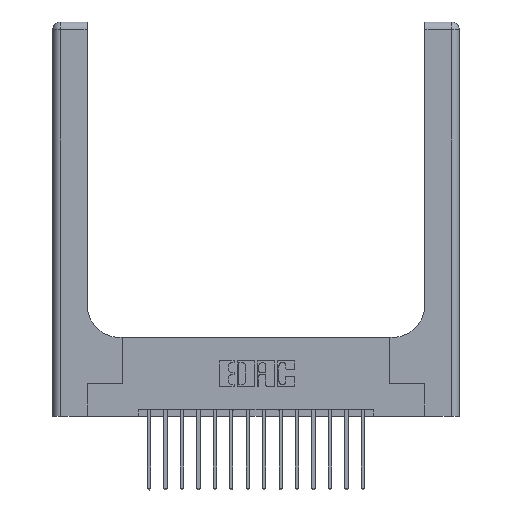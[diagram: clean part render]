
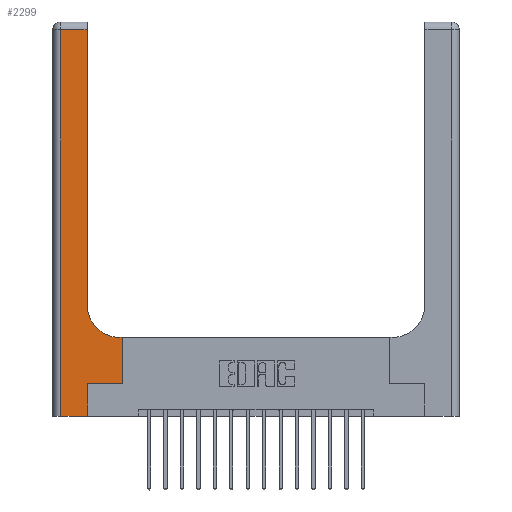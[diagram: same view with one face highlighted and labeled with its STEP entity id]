
A CAD part, top view. The second image highlights one B-rep face of the part: STEP entity #2299.
In plain terms, the highlighted planar face has unit normal (0, 0, 1).
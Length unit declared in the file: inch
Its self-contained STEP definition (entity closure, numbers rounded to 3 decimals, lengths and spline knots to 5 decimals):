
#27 = VERTEX_POINT ( 'NONE', #10364 ) ;
#259 = VERTEX_POINT ( 'NONE', #10660 ) ;
#442 = VECTOR ( 'NONE', #9737, 39.37008 ) ;
#500 = DIRECTION ( 'NONE',  ( 0., 1., 0. ) ) ;
#886 = CARTESIAN_POINT ( 'NONE',  ( 0.528, 0.25, 0.37 ) ) ;
#1867 = VERTEX_POINT ( 'NONE', #3295 ) ;
#1930 = VECTOR ( 'NONE', #9675, 39.37008 ) ;
#2299 = ADVANCED_FACE ( 'NONE', ( #17613 ), #8410, .F. ) ;
#2302 = ORIENTED_EDGE ( 'NONE', *, *, #12450, .T. ) ;
#2463 = CARTESIAN_POINT ( 'NONE',  ( 0., 0., 0.37 ) ) ;
#2522 = EDGE_CURVE ( 'NONE', #1867, #12474, #10802, .T. ) ;
#2961 = VECTOR ( 'NONE', #17435, 39.37008 ) ;
#3037 = ORIENTED_EDGE ( 'NONE', *, *, #3047, .T. ) ;
#3047 = EDGE_CURVE ( 'NONE', #12474, #259, #11000, .T. ) ;
#3295 = CARTESIAN_POINT ( 'NONE',  ( 0.528, 0.25, 0.37 ) ) ;
#3488 = ORIENTED_EDGE ( 'NONE', *, *, #9466, .T. ) ;
#3636 = DIRECTION ( 'NONE',  ( 1., 0., 0. ) ) ;
#3998 = AXIS2_PLACEMENT_3D ( 'NONE', #11201, #16624, #9816 ) ;
#4140 = ORIENTED_EDGE ( 'NONE', *, *, #8069, .T. ) ;
#4178 = CARTESIAN_POINT ( 'NONE',  ( 0.265, 0., 0.37 ) ) ;
#4180 = CARTESIAN_POINT ( 'NONE',  ( 0.265, 0.25, 0.37 ) ) ;
#4676 = ORIENTED_EDGE ( 'NONE', *, *, #7464, .T. ) ;
#4763 = LINE ( 'NONE', #4180, #16792 ) ;
#4932 = CARTESIAN_POINT ( 'NONE',  ( 0.51, 0.85, 0.37 ) ) ;
#5032 = CARTESIAN_POINT ( 'NONE',  ( 0.06, 2.94, 0.37 ) ) ;
#5108 = DIRECTION ( 'NONE',  ( 1., 0., 0. ) ) ;
#6316 = EDGE_CURVE ( 'NONE', #13782, #11043, #7664, .T. ) ;
#6340 = DIRECTION ( 'NONE',  ( 0., 0., -1. ) ) ;
#6595 = ORIENTED_EDGE ( 'NONE', *, *, #8855, .T. ) ;
#7026 = VERTEX_POINT ( 'NONE', #9818 ) ;
#7166 = LINE ( 'NONE', #11311, #1930 ) ;
#7381 = VECTOR ( 'NONE', #13764, 39.37008 ) ;
#7464 = EDGE_CURVE ( 'NONE', #11043, #27, #16376, .T. ) ;
#7519 = ORIENTED_EDGE ( 'NONE', *, *, #17191, .T. ) ;
#7664 = LINE ( 'NONE', #2463, #10480 ) ;
#8069 = EDGE_CURVE ( 'NONE', #7026, #16161, #7166, .T. ) ;
#8212 = ORIENTED_EDGE ( 'NONE', *, *, #2522, .T. ) ;
#8323 = DIRECTION ( 'NONE',  ( -1., 0., 0. ) ) ;
#8410 = PLANE ( 'NONE',  #3998 ) ;
#8855 = EDGE_CURVE ( 'NONE', #27, #1867, #4763, .T. ) ;
#9466 = EDGE_CURVE ( 'NONE', #16161, #13782, #15250, .T. ) ;
#9675 = DIRECTION ( 'NONE',  ( -1., 0., 0. ) ) ;
#9737 = DIRECTION ( 'NONE',  ( 0., 1., 0. ) ) ;
#9796 = ORIENTED_EDGE ( 'NONE', *, *, #6316, .T. ) ;
#9816 = DIRECTION ( 'NONE',  ( -1., 0., 0. ) ) ;
#9818 = CARTESIAN_POINT ( 'NONE',  ( 0.26, 2.94, 0.37 ) ) ;
#10044 = CARTESIAN_POINT ( 'NONE',  ( 0.528, 0.6, 0.37 ) ) ;
#10364 = CARTESIAN_POINT ( 'NONE',  ( 0.265, 0.25, 0.37 ) ) ;
#10480 = VECTOR ( 'NONE', #5108, 39.37008 ) ;
#10660 = CARTESIAN_POINT ( 'NONE',  ( 0.51, 0.6, 0.37 ) ) ;
#10802 = LINE ( 'NONE', #886, #2961 ) ;
#11000 = LINE ( 'NONE', #14005, #17596 ) ;
#11043 = VERTEX_POINT ( 'NONE', #4178 ) ;
#11201 = CARTESIAN_POINT ( 'NONE',  ( 0., 3., 0.37 ) ) ;
#11311 = CARTESIAN_POINT ( 'NONE',  ( 0., 2.94, 0.37 ) ) ;
#12450 = EDGE_CURVE ( 'NONE', #13371, #7026, #14671, .T. ) ;
#12474 = VERTEX_POINT ( 'NONE', #10044 ) ;
#12626 = VECTOR ( 'NONE', #500, 39.37008 ) ;
#12689 = AXIS2_PLACEMENT_3D ( 'NONE', #4932, #6340, #3636 ) ;
#13371 = VERTEX_POINT ( 'NONE', #13662 ) ;
#13662 = CARTESIAN_POINT ( 'NONE',  ( 0.26, 0.85, 0.37 ) ) ;
#13764 = DIRECTION ( 'NONE',  ( 0., -1., 0. ) ) ;
#13782 = VERTEX_POINT ( 'NONE', #15871 ) ;
#13957 = DIRECTION ( 'NONE',  ( 1., 0., 0. ) ) ;
#14005 = CARTESIAN_POINT ( 'NONE',  ( 0.26, 0.6, 0.37 ) ) ;
#14253 = CARTESIAN_POINT ( 'NONE',  ( 0.265, 0., 0.37 ) ) ;
#14671 = LINE ( 'NONE', #15370, #442 ) ;
#14719 = CIRCLE ( 'NONE', #12689, 0.25 ) ;
#15234 = CARTESIAN_POINT ( 'NONE',  ( 0.06, 3., 0.37 ) ) ;
#15250 = LINE ( 'NONE', #15234, #7381 ) ;
#15370 = CARTESIAN_POINT ( 'NONE',  ( 0.26, 3., 0.37 ) ) ;
#15871 = CARTESIAN_POINT ( 'NONE',  ( 0.06, 0., 0.37 ) ) ;
#15872 = EDGE_LOOP ( 'NONE', ( #2302, #4140, #3488, #9796, #4676, #6595, #8212, #3037, #7519 ) ) ;
#16161 = VERTEX_POINT ( 'NONE', #5032 ) ;
#16376 = LINE ( 'NONE', #14253, #12626 ) ;
#16624 = DIRECTION ( 'NONE',  ( 0., 0., -1. ) ) ;
#16792 = VECTOR ( 'NONE', #13957, 39.37008 ) ;
#17191 = EDGE_CURVE ( 'NONE', #259, #13371, #14719, .T. ) ;
#17435 = DIRECTION ( 'NONE',  ( 0., 1., 0. ) ) ;
#17596 = VECTOR ( 'NONE', #8323, 39.37008 ) ;
#17613 = FACE_OUTER_BOUND ( 'NONE', #15872, .T. ) ;
